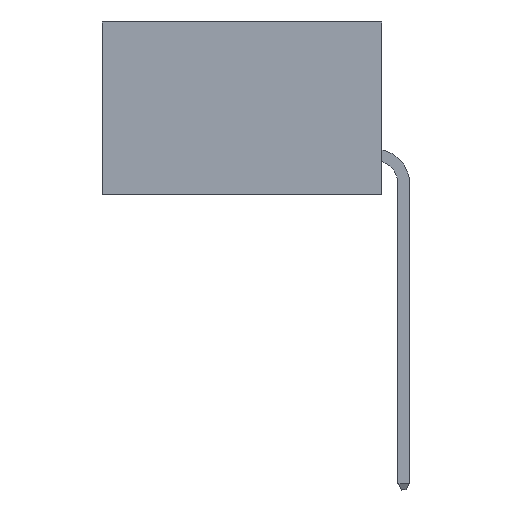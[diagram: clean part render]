
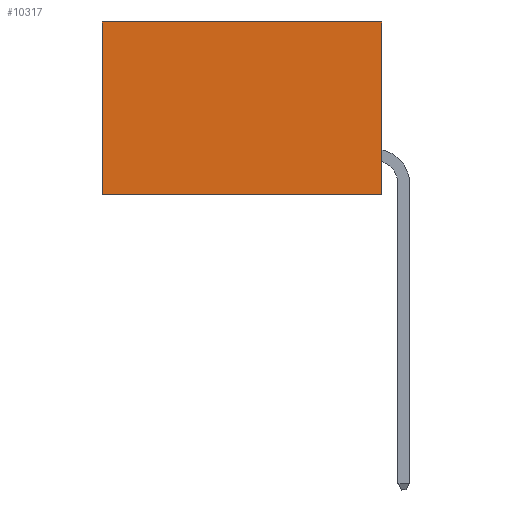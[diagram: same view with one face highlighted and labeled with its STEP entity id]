
A CAD part, left-side view. The second image highlights one B-rep face of the part: STEP entity #10317.
In plain terms, the highlighted planar face has unit normal (-1, 0, 0).
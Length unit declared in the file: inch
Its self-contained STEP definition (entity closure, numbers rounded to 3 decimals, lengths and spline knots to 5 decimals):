
#845 = CARTESIAN_POINT ( 'NONE',  ( 0.2875, 0., 0. ) ) ;
#951 = VERTEX_POINT ( 'NONE', #26218 ) ;
#1563 = EDGE_CURVE ( 'NONE', #5113, #25559, #29011, .T. ) ;
#2333 = CARTESIAN_POINT ( 'NONE',  ( 0.2875, 0.6, -0.37 ) ) ;
#2431 = EDGE_LOOP ( 'NONE', ( #8561, #33350, #6635, #6877 ) ) ;
#3996 = CARTESIAN_POINT ( 'NONE',  ( 0.2875, 0.6, 0. ) ) ;
#4085 = DIRECTION ( 'NONE',  ( 0., 0., -1. ) ) ;
#5113 = VERTEX_POINT ( 'NONE', #38593 ) ;
#5207 = VECTOR ( 'NONE', #16577, 39.37008 ) ;
#6635 = ORIENTED_EDGE ( 'NONE', *, *, #37665, .F. ) ;
#6877 = ORIENTED_EDGE ( 'NONE', *, *, #31911, .T. ) ;
#7309 = CARTESIAN_POINT ( 'NONE',  ( 0.2875, 0., 0. ) ) ;
#7397 = VECTOR ( 'NONE', #22441, 39.37008 ) ;
#8561 = ORIENTED_EDGE ( 'NONE', *, *, #38232, .T. ) ;
#10317 = ADVANCED_FACE ( 'NONE', ( #24669 ), #39600, .F. ) ;
#15498 = VECTOR ( 'NONE', #17337, 39.37008 ) ;
#16577 = DIRECTION ( 'NONE',  ( 0., 0., -1. ) ) ;
#17337 = DIRECTION ( 'NONE',  ( 0., 1., 0. ) ) ;
#19689 = CARTESIAN_POINT ( 'NONE',  ( 0.2875, 0., 0. ) ) ;
#19879 = LINE ( 'NONE', #19689, #5207 ) ;
#20334 = VERTEX_POINT ( 'NONE', #35661 ) ;
#22441 = DIRECTION ( 'NONE',  ( 0., 1., 0. ) ) ;
#24590 = LINE ( 'NONE', #845, #15498 ) ;
#24669 = FACE_OUTER_BOUND ( 'NONE', #2431, .T. ) ;
#25559 = VERTEX_POINT ( 'NONE', #2333 ) ;
#26218 = CARTESIAN_POINT ( 'NONE',  ( 0.2875, 0.6, 0. ) ) ;
#27393 = AXIS2_PLACEMENT_3D ( 'NONE', #7309, #32776, #4085 ) ;
#28807 = LINE ( 'NONE', #3996, #40991 ) ;
#29011 = LINE ( 'NONE', #38749, #7397 ) ;
#31911 = EDGE_CURVE ( 'NONE', #20334, #951, #24590, .T. ) ;
#32776 = DIRECTION ( 'NONE',  ( 1., 0., 0. ) ) ;
#33350 = ORIENTED_EDGE ( 'NONE', *, *, #1563, .F. ) ;
#33508 = DIRECTION ( 'NONE',  ( 0., 0., -1. ) ) ;
#35661 = CARTESIAN_POINT ( 'NONE',  ( 0.2875, 0., 0. ) ) ;
#37665 = EDGE_CURVE ( 'NONE', #20334, #5113, #19879, .T. ) ;
#38232 = EDGE_CURVE ( 'NONE', #951, #25559, #28807, .T. ) ;
#38593 = CARTESIAN_POINT ( 'NONE',  ( 0.2875, 0., -0.37 ) ) ;
#38749 = CARTESIAN_POINT ( 'NONE',  ( 0.2875, 0., -0.37 ) ) ;
#39600 = PLANE ( 'NONE',  #27393 ) ;
#40991 = VECTOR ( 'NONE', #33508, 39.37008 ) ;
